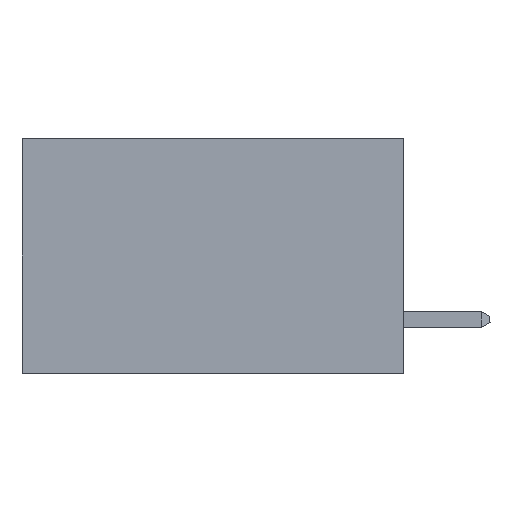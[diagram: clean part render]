
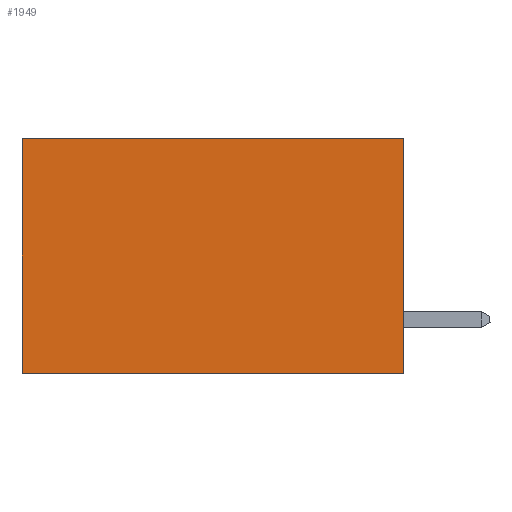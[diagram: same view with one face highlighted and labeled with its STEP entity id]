
A CAD part, left-side view. The second image highlights one B-rep face of the part: STEP entity #1949.
In plain terms, the highlighted planar face has unit normal (-1, 0, 0).
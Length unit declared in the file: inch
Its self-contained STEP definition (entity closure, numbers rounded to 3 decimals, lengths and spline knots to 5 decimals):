
#195 = VERTEX_POINT ( 'NONE', #3862 ) ;
#209 = PLANE ( 'NONE',  #5690 ) ;
#1067 = LINE ( 'NONE', #8495, #10856 ) ;
#1088 = VERTEX_POINT ( 'NONE', #4071 ) ;
#1949 = ADVANCED_FACE ( 'NONE', ( #12540 ), #209, .F. ) ;
#2183 = ORIENTED_EDGE ( 'NONE', *, *, #7033, .F. ) ;
#2226 = DIRECTION ( 'NONE',  ( 1., 0., 0. ) ) ;
#2574 = VERTEX_POINT ( 'NONE', #2928 ) ;
#2846 = CARTESIAN_POINT ( 'NONE',  ( 0.2875, 0.6, 0. ) ) ;
#2928 = CARTESIAN_POINT ( 'NONE',  ( 0.2875, 0.6, 0. ) ) ;
#3230 = DIRECTION ( 'NONE',  ( 0., 0., -1. ) ) ;
#3555 = CARTESIAN_POINT ( 'NONE',  ( 0.2875, 0., -0.37 ) ) ;
#3848 = EDGE_CURVE ( 'NONE', #1088, #2574, #4568, .T. ) ;
#3862 = CARTESIAN_POINT ( 'NONE',  ( 0.2875, 0.6, -0.37 ) ) ;
#4071 = CARTESIAN_POINT ( 'NONE',  ( 0.2875, 0., 0. ) ) ;
#4178 = CARTESIAN_POINT ( 'NONE',  ( 0.2875, 0., 0. ) ) ;
#4390 = DIRECTION ( 'NONE',  ( 0., 1., 0. ) ) ;
#4568 = LINE ( 'NONE', #4178, #10779 ) ;
#4664 = ORIENTED_EDGE ( 'NONE', *, *, #11665, .F. ) ;
#5690 = AXIS2_PLACEMENT_3D ( 'NONE', #10160, #2226, #3230 ) ;
#6236 = ORIENTED_EDGE ( 'NONE', *, *, #3848, .T. ) ;
#6331 = EDGE_LOOP ( 'NONE', ( #8619, #2183, #4664, #6236 ) ) ;
#6336 = DIRECTION ( 'NONE',  ( 0., 1., 0. ) ) ;
#6441 = EDGE_CURVE ( 'NONE', #2574, #195, #12692, .T. ) ;
#6529 = VECTOR ( 'NONE', #8596, 39.37008 ) ;
#6658 = CARTESIAN_POINT ( 'NONE',  ( 0.2875, 0., 0. ) ) ;
#6673 = VECTOR ( 'NONE', #10890, 39.37008 ) ;
#7033 = EDGE_CURVE ( 'NONE', #8829, #195, #1067, .T. ) ;
#8495 = CARTESIAN_POINT ( 'NONE',  ( 0.2875, 0., -0.37 ) ) ;
#8596 = DIRECTION ( 'NONE',  ( 0., 0., -1. ) ) ;
#8619 = ORIENTED_EDGE ( 'NONE', *, *, #6441, .T. ) ;
#8829 = VERTEX_POINT ( 'NONE', #3555 ) ;
#9210 = LINE ( 'NONE', #6658, #6529 ) ;
#10160 = CARTESIAN_POINT ( 'NONE',  ( 0.2875, 0., 0. ) ) ;
#10779 = VECTOR ( 'NONE', #4390, 39.37008 ) ;
#10856 = VECTOR ( 'NONE', #6336, 39.37008 ) ;
#10890 = DIRECTION ( 'NONE',  ( 0., 0., -1. ) ) ;
#11665 = EDGE_CURVE ( 'NONE', #1088, #8829, #9210, .T. ) ;
#12540 = FACE_OUTER_BOUND ( 'NONE', #6331, .T. ) ;
#12692 = LINE ( 'NONE', #2846, #6673 ) ;
